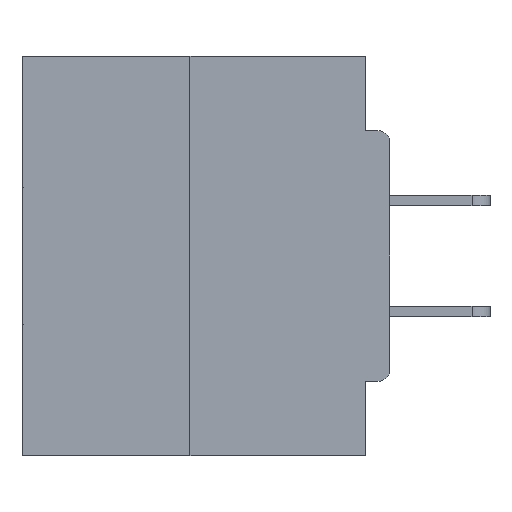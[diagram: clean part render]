
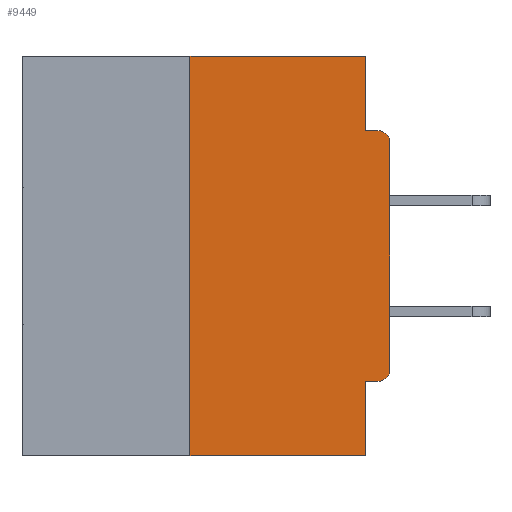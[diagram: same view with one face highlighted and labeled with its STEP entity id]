
A CAD part, left-side view. The second image highlights one B-rep face of the part: STEP entity #9449.
In plain terms, the highlighted planar face has unit normal (-1, 0, 0).
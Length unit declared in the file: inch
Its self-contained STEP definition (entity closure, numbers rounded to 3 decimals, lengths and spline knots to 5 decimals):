
#804 = VERTEX_POINT ( 'NONE', #17757 ) ;
#1122 = VERTEX_POINT ( 'NONE', #31664 ) ;
#1640 = ORIENTED_EDGE ( 'NONE', *, *, #29351, .F. ) ;
#1708 = CARTESIAN_POINT ( 'NONE',  ( 0., 0.031, 0. ) ) ;
#2482 = LINE ( 'NONE', #30357, #22907 ) ;
#2629 = LINE ( 'NONE', #31874, #26208 ) ;
#2926 = VECTOR ( 'NONE', #18212, 39.37008 ) ;
#3025 = AXIS2_PLACEMENT_3D ( 'NONE', #31558, #31437, #14029 ) ;
#3055 = VECTOR ( 'NONE', #19362, 39.37008 ) ;
#4000 = EDGE_CURVE ( 'NONE', #804, #29050, #34879, .T. ) ;
#5122 = EDGE_CURVE ( 'NONE', #17099, #6086, #2482, .T. ) ;
#6086 = VERTEX_POINT ( 'NONE', #19571 ) ;
#6214 = VERTEX_POINT ( 'NONE', #16427 ) ;
#8099 = FACE_OUTER_BOUND ( 'NONE', #11425, .T. ) ;
#8804 = VERTEX_POINT ( 'NONE', #19671 ) ;
#9047 = ORIENTED_EDGE ( 'NONE', *, *, #28004, .F. ) ;
#9449 = ADVANCED_FACE ( 'NONE', ( #8099 ), #13815, .F. ) ;
#9608 = LINE ( 'NONE', #32772, #35998 ) ;
#9644 = EDGE_CURVE ( 'NONE', #1122, #17590, #2629, .T. ) ;
#9741 = DIRECTION ( 'NONE',  ( 0., 0., 1. ) ) ;
#9817 = CIRCLE ( 'NONE', #25090, 0.015 ) ;
#10431 = EDGE_CURVE ( 'NONE', #31074, #8804, #9817, .T. ) ;
#10535 = DIRECTION ( 'NONE',  ( 1., 0., 0. ) ) ;
#11009 = AXIS2_PLACEMENT_3D ( 'NONE', #31237, #10535, #16610 ) ;
#11425 = EDGE_LOOP ( 'NONE', ( #9047, #20510, #35579, #14879, #19132, #21653, #32288, #13979, #1640, #20064 ) ) ;
#13815 = PLANE ( 'NONE',  #11009 ) ;
#13979 = ORIENTED_EDGE ( 'NONE', *, *, #10431, .T. ) ;
#14029 = DIRECTION ( 'NONE',  ( 0., 0., -1. ) ) ;
#14879 = ORIENTED_EDGE ( 'NONE', *, *, #21251, .F. ) ;
#15446 = CARTESIAN_POINT ( 'NONE',  ( 0., 0.25, 0. ) ) ;
#16306 = CARTESIAN_POINT ( 'NONE',  ( 0., 0.031, -0.4065 ) ) ;
#16361 = CARTESIAN_POINT ( 'NONE',  ( 0., 0.015, -0.1085 ) ) ;
#16427 = CARTESIAN_POINT ( 'NONE',  ( 0., 0., -0.3915 ) ) ;
#16610 = DIRECTION ( 'NONE',  ( 0., 0., -1. ) ) ;
#16899 = DIRECTION ( 'NONE',  ( 0., -1., 0. ) ) ;
#16942 = VERTEX_POINT ( 'NONE', #18748 ) ;
#17099 = VERTEX_POINT ( 'NONE', #1708 ) ;
#17590 = VERTEX_POINT ( 'NONE', #15446 ) ;
#17699 = CARTESIAN_POINT ( 'NONE',  ( 0., 0., 0. ) ) ;
#17757 = CARTESIAN_POINT ( 'NONE',  ( 0., 0.015, -0.4065 ) ) ;
#18212 = DIRECTION ( 'NONE',  ( 0., 0., 1. ) ) ;
#18748 = CARTESIAN_POINT ( 'NONE',  ( 0., 0.031, -0.5 ) ) ;
#19132 = ORIENTED_EDGE ( 'NONE', *, *, #4000, .F. ) ;
#19362 = DIRECTION ( 'NONE',  ( 0., 1., 0. ) ) ;
#19571 = CARTESIAN_POINT ( 'NONE',  ( 0., 0.031, -0.0935 ) ) ;
#19671 = CARTESIAN_POINT ( 'NONE',  ( 0., 0.015, -0.0935 ) ) ;
#20064 = ORIENTED_EDGE ( 'NONE', *, *, #5122, .F. ) ;
#20510 = ORIENTED_EDGE ( 'NONE', *, *, #9644, .F. ) ;
#21128 = CARTESIAN_POINT ( 'NONE',  ( 0., 0.46, -0.5 ) ) ;
#21251 = EDGE_CURVE ( 'NONE', #29050, #16942, #9608, .T. ) ;
#21557 = LINE ( 'NONE', #17699, #2926 ) ;
#21653 = ORIENTED_EDGE ( 'NONE', *, *, #31371, .T. ) ;
#21701 = DIRECTION ( 'NONE',  ( 0., 0., -1. ) ) ;
#22198 = DIRECTION ( 'NONE',  ( 0., 0., -1. ) ) ;
#22907 = VECTOR ( 'NONE', #21701, 39.37008 ) ;
#23352 = VECTOR ( 'NONE', #37061, 39.37008 ) ;
#25004 = LINE ( 'NONE', #21128, #31431 ) ;
#25063 = VECTOR ( 'NONE', #16899, 39.37008 ) ;
#25090 = AXIS2_PLACEMENT_3D ( 'NONE', #16361, #28184, #22198 ) ;
#25283 = CARTESIAN_POINT ( 'NONE',  ( 0., 0., -0.4065 ) ) ;
#26208 = VECTOR ( 'NONE', #9741, 39.37008 ) ;
#27057 = DIRECTION ( 'NONE',  ( 0., -1., 0. ) ) ;
#28004 = EDGE_CURVE ( 'NONE', #17590, #17099, #35232, .T. ) ;
#28184 = DIRECTION ( 'NONE',  ( -1., 0., 0. ) ) ;
#28336 = EDGE_CURVE ( 'NONE', #6214, #31074, #21557, .T. ) ;
#28479 = CARTESIAN_POINT ( 'NONE',  ( 0., 0., -0.0935 ) ) ;
#29050 = VERTEX_POINT ( 'NONE', #16306 ) ;
#29351 = EDGE_CURVE ( 'NONE', #6086, #8804, #30567, .T. ) ;
#29634 = CIRCLE ( 'NONE', #3025, 0.015 ) ;
#30357 = CARTESIAN_POINT ( 'NONE',  ( 0., 0.031, 0. ) ) ;
#30567 = LINE ( 'NONE', #28479, #25063 ) ;
#31074 = VERTEX_POINT ( 'NONE', #32998 ) ;
#31237 = CARTESIAN_POINT ( 'NONE',  ( 0., 0.46, 0. ) ) ;
#31371 = EDGE_CURVE ( 'NONE', #804, #6214, #29634, .T. ) ;
#31431 = VECTOR ( 'NONE', #27057, 39.37008 ) ;
#31437 = DIRECTION ( 'NONE',  ( -1., 0., 0. ) ) ;
#31449 = EDGE_CURVE ( 'NONE', #1122, #16942, #25004, .T. ) ;
#31558 = CARTESIAN_POINT ( 'NONE',  ( 0., 0.015, -0.3915 ) ) ;
#31664 = CARTESIAN_POINT ( 'NONE',  ( 0., 0.25, -0.5 ) ) ;
#31874 = CARTESIAN_POINT ( 'NONE',  ( 0., 0.25, 0. ) ) ;
#32288 = ORIENTED_EDGE ( 'NONE', *, *, #28336, .T. ) ;
#32772 = CARTESIAN_POINT ( 'NONE',  ( 0., 0.031, -0.5 ) ) ;
#32998 = CARTESIAN_POINT ( 'NONE',  ( 0., 0., -0.1085 ) ) ;
#34879 = LINE ( 'NONE', #25283, #3055 ) ;
#35232 = LINE ( 'NONE', #36929, #23352 ) ;
#35579 = ORIENTED_EDGE ( 'NONE', *, *, #31449, .T. ) ;
#35959 = DIRECTION ( 'NONE',  ( 0., 0., -1. ) ) ;
#35998 = VECTOR ( 'NONE', #35959, 39.37008 ) ;
#36929 = CARTESIAN_POINT ( 'NONE',  ( 0., 0.46, 0. ) ) ;
#37061 = DIRECTION ( 'NONE',  ( 0., -1., 0. ) ) ;
